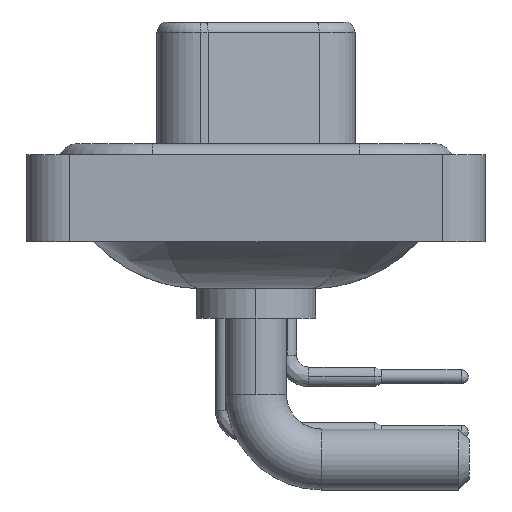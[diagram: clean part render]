
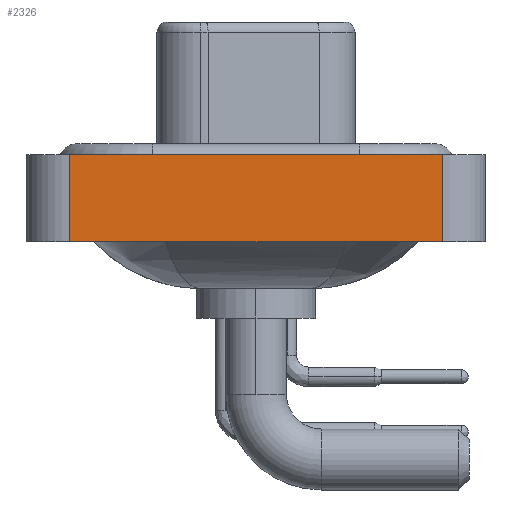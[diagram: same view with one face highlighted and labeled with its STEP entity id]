
A CAD part, left-side view. The second image highlights one B-rep face of the part: STEP entity #2326.
In plain terms, the highlighted planar face has unit normal (-1, 0, 0).
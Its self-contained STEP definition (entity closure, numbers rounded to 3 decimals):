
#734 = LINE ( 'NONE', #6428, #8436 ) ;
#981 = EDGE_CURVE ( 'NONE', #15099, #2747, #8236, .T. ) ;
#1091 = LINE ( 'NONE', #22111, #14660 ) ;
#1425 = DIRECTION ( 'NONE',  ( 0., 0., 1. ) ) ;
#1548 = FACE_OUTER_BOUND ( 'NONE', #4795, .T. ) ;
#2120 = CARTESIAN_POINT ( 'NONE',  ( -7.3, -8.55, -3.6 ) ) ;
#2326 = ADVANCED_FACE ( 'NONE', ( #1548 ), #12834, .T. ) ;
#2625 = VECTOR ( 'NONE', #13724, 1000. ) ;
#2747 = VERTEX_POINT ( 'NONE', #16926 ) ;
#4795 = EDGE_LOOP ( 'NONE', ( #12502, #19533, #21574, #10772 ) ) ;
#4920 = DIRECTION ( 'NONE',  ( 0., -1., 0. ) ) ;
#6428 = CARTESIAN_POINT ( 'NONE',  ( -7.3, 8.55, -3.6 ) ) ;
#6617 = EDGE_CURVE ( 'NONE', #12449, #15099, #734, .T. ) ;
#6988 = DIRECTION ( 'NONE',  ( -1., 0., 0. ) ) ;
#8236 = LINE ( 'NONE', #19814, #2625 ) ;
#8436 = VECTOR ( 'NONE', #18142, 1000. ) ;
#10772 = ORIENTED_EDGE ( 'NONE', *, *, #17152, .T. ) ;
#10823 = VERTEX_POINT ( 'NONE', #2120 ) ;
#12449 = VERTEX_POINT ( 'NONE', #20158 ) ;
#12502 = ORIENTED_EDGE ( 'NONE', *, *, #13264, .T. ) ;
#12834 = PLANE ( 'NONE',  #17039 ) ;
#13237 = VECTOR ( 'NONE', #20193, 1000. ) ;
#13264 = EDGE_CURVE ( 'NONE', #10823, #2747, #18587, .T. ) ;
#13724 = DIRECTION ( 'NONE',  ( 0., -1., 0. ) ) ;
#14660 = VECTOR ( 'NONE', #4920, 1000. ) ;
#15099 = VERTEX_POINT ( 'NONE', #18459 ) ;
#16926 = CARTESIAN_POINT ( 'NONE',  ( -7.3, -8.55, 0.4 ) ) ;
#17039 = AXIS2_PLACEMENT_3D ( 'NONE', #24037, #6988, #1425 ) ;
#17152 = EDGE_CURVE ( 'NONE', #12449, #10823, #1091, .T. ) ;
#18142 = DIRECTION ( 'NONE',  ( 0., 0., 1. ) ) ;
#18459 = CARTESIAN_POINT ( 'NONE',  ( -7.3, 8.55, 0.4 ) ) ;
#18587 = LINE ( 'NONE', #23807, #13237 ) ;
#19533 = ORIENTED_EDGE ( 'NONE', *, *, #981, .F. ) ;
#19814 = CARTESIAN_POINT ( 'NONE',  ( -7.3, -8.55, 0.4 ) ) ;
#20158 = CARTESIAN_POINT ( 'NONE',  ( -7.3, 8.55, -3.6 ) ) ;
#20193 = DIRECTION ( 'NONE',  ( 0., 0., 1. ) ) ;
#21574 = ORIENTED_EDGE ( 'NONE', *, *, #6617, .F. ) ;
#22111 = CARTESIAN_POINT ( 'NONE',  ( -7.3, -8.55, -3.6 ) ) ;
#23807 = CARTESIAN_POINT ( 'NONE',  ( -7.3, -8.55, -3.6 ) ) ;
#24037 = CARTESIAN_POINT ( 'NONE',  ( -7.3, -8.55, -3.6 ) ) ;
